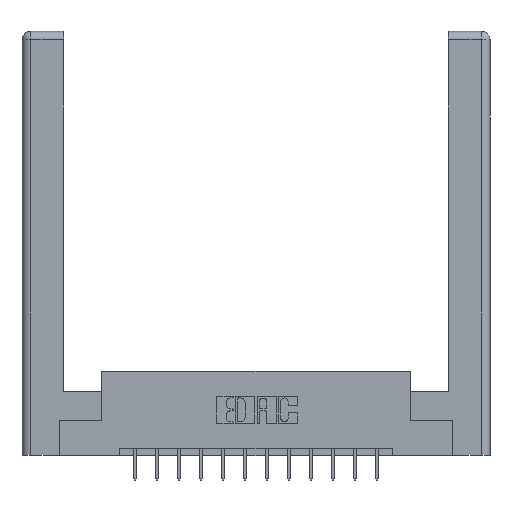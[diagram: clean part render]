
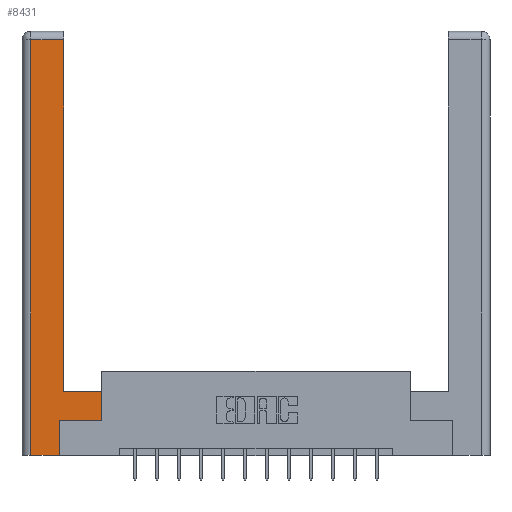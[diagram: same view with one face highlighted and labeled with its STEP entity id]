
A CAD part, top view. The second image highlights one B-rep face of the part: STEP entity #8431.
In plain terms, the highlighted planar face has unit normal (0, 0, 1).
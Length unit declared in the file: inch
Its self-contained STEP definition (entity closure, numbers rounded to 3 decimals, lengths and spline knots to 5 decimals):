
#139 = ORIENTED_EDGE ( 'NONE', *, *, #734, .T. ) ;
#320 = DIRECTION ( 'NONE',  ( 0., 1., 0. ) ) ;
#604 = VECTOR ( 'NONE', #11035, 39.37008 ) ;
#734 = EDGE_CURVE ( 'NONE', #1591, #1885, #11576, .T. ) ;
#812 = EDGE_LOOP ( 'NONE', ( #4407, #822, #13347, #4381, #8551, #2618, #13770, #139 ) ) ;
#822 = ORIENTED_EDGE ( 'NONE', *, *, #2528, .T. ) ;
#1127 = EDGE_CURVE ( 'NONE', #15290, #3762, #2491, .T. ) ;
#1191 = CARTESIAN_POINT ( 'NONE',  ( 0.565, 0.245, 0. ) ) ;
#1336 = CARTESIAN_POINT ( 'NONE',  ( 0.565, 0.45, 0. ) ) ;
#1423 = EDGE_CURVE ( 'NONE', #1885, #9357, #6122, .T. ) ;
#1435 = LINE ( 'NONE', #14068, #9903 ) ;
#1591 = VERTEX_POINT ( 'NONE', #1336 ) ;
#1760 = VECTOR ( 'NONE', #5726, 39.37008 ) ;
#1799 = EDGE_CURVE ( 'NONE', #14670, #3551, #4528, .T. ) ;
#1885 = VERTEX_POINT ( 'NONE', #4789 ) ;
#2491 = LINE ( 'NONE', #4687, #15580 ) ;
#2528 = EDGE_CURVE ( 'NONE', #9357, #7005, #1435, .T. ) ;
#2570 = CARTESIAN_POINT ( 'NONE',  ( 0.295, 2.94, 0. ) ) ;
#2618 = ORIENTED_EDGE ( 'NONE', *, *, #1799, .T. ) ;
#3551 = VERTEX_POINT ( 'NONE', #4449 ) ;
#3762 = VERTEX_POINT ( 'NONE', #12494 ) ;
#3952 = CARTESIAN_POINT ( 'NONE',  ( 0.295, 3., 0. ) ) ;
#4381 = ORIENTED_EDGE ( 'NONE', *, *, #1127, .T. ) ;
#4383 = DIRECTION ( 'NONE',  ( 0., 0., -1. ) ) ;
#4407 = ORIENTED_EDGE ( 'NONE', *, *, #1423, .T. ) ;
#4449 = CARTESIAN_POINT ( 'NONE',  ( 0.565, 0.245, 0. ) ) ;
#4528 = LINE ( 'NONE', #1191, #6248 ) ;
#4687 = CARTESIAN_POINT ( 'NONE',  ( 0.265, 0., 0. ) ) ;
#4781 = DIRECTION ( 'NONE',  ( 1., 0., 0. ) ) ;
#4789 = CARTESIAN_POINT ( 'NONE',  ( 0.295, 0.45, 0. ) ) ;
#5368 = VECTOR ( 'NONE', #320, 39.37008 ) ;
#5726 = DIRECTION ( 'NONE',  ( 0., 1., 0. ) ) ;
#5996 = CARTESIAN_POINT ( 'NONE',  ( 0.0615, 0., 0. ) ) ;
#6122 = LINE ( 'NONE', #3952, #5368 ) ;
#6243 = DIRECTION ( 'NONE',  ( 1., 0., 0. ) ) ;
#6248 = VECTOR ( 'NONE', #6243, 39.37008 ) ;
#6398 = DIRECTION ( 'NONE',  ( 0., 1., 0. ) ) ;
#6545 = LINE ( 'NONE', #6846, #1760 ) ;
#6846 = CARTESIAN_POINT ( 'NONE',  ( 0.565, 0.45, 0. ) ) ;
#7002 = CARTESIAN_POINT ( 'NONE',  ( 0.0615, 0., 0. ) ) ;
#7005 = VERTEX_POINT ( 'NONE', #11911 ) ;
#7402 = FACE_OUTER_BOUND ( 'NONE', #812, .T. ) ;
#8431 = ADVANCED_FACE ( 'NONE', ( #7402 ), #9408, .F. ) ;
#8551 = ORIENTED_EDGE ( 'NONE', *, *, #9857, .T. ) ;
#9105 = LINE ( 'NONE', #11552, #13867 ) ;
#9357 = VERTEX_POINT ( 'NONE', #2570 ) ;
#9363 = DIRECTION ( 'NONE',  ( -1., 0., 0. ) ) ;
#9408 = PLANE ( 'NONE',  #12493 ) ;
#9857 = EDGE_CURVE ( 'NONE', #3762, #14670, #9105, .T. ) ;
#9903 = VECTOR ( 'NONE', #9363, 39.37008 ) ;
#10488 = DIRECTION ( 'NONE',  ( -1., 0., 0. ) ) ;
#10699 = EDGE_CURVE ( 'NONE', #3551, #1591, #6545, .T. ) ;
#11035 = DIRECTION ( 'NONE',  ( 0., -1., 0. ) ) ;
#11183 = LINE ( 'NONE', #5996, #604 ) ;
#11437 = EDGE_CURVE ( 'NONE', #7005, #15290, #11183, .T. ) ;
#11552 = CARTESIAN_POINT ( 'NONE',  ( 0.265, 0.245, 0. ) ) ;
#11576 = LINE ( 'NONE', #15202, #14420 ) ;
#11911 = CARTESIAN_POINT ( 'NONE',  ( 0.0615, 2.94, 0. ) ) ;
#12106 = CARTESIAN_POINT ( 'NONE',  ( 0.265, 0.245, 0. ) ) ;
#12493 = AXIS2_PLACEMENT_3D ( 'NONE', #15468, #4383, #10488 ) ;
#12494 = CARTESIAN_POINT ( 'NONE',  ( 0.265, 0., 0. ) ) ;
#13347 = ORIENTED_EDGE ( 'NONE', *, *, #11437, .T. ) ;
#13770 = ORIENTED_EDGE ( 'NONE', *, *, #10699, .T. ) ;
#13867 = VECTOR ( 'NONE', #6398, 39.37008 ) ;
#14068 = CARTESIAN_POINT ( 'NONE',  ( 0.0615, 2.94, 0. ) ) ;
#14420 = VECTOR ( 'NONE', #14989, 39.37008 ) ;
#14670 = VERTEX_POINT ( 'NONE', #12106 ) ;
#14989 = DIRECTION ( 'NONE',  ( -1., 0., 0. ) ) ;
#15202 = CARTESIAN_POINT ( 'NONE',  ( 0.295, 0.45, 0. ) ) ;
#15290 = VERTEX_POINT ( 'NONE', #7002 ) ;
#15468 = CARTESIAN_POINT ( 'NONE',  ( 0., 0., 0. ) ) ;
#15580 = VECTOR ( 'NONE', #4781, 39.37008 ) ;
